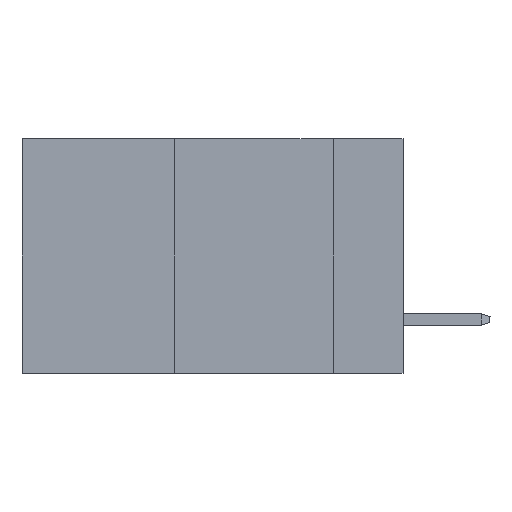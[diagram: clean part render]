
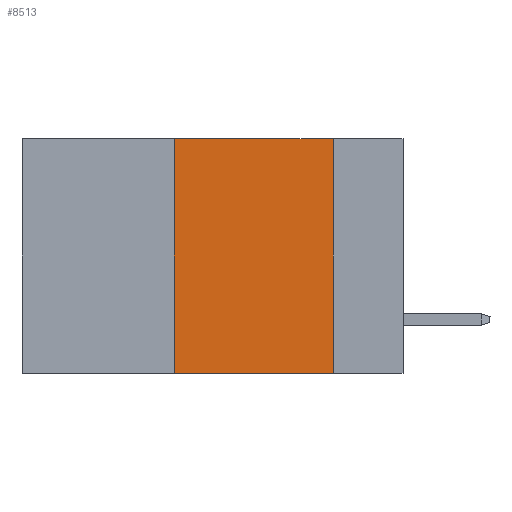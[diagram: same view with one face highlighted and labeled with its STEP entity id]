
A CAD part, left-side view. The second image highlights one B-rep face of the part: STEP entity #8513.
In plain terms, the highlighted planar face has unit normal (-1, 0, 0).
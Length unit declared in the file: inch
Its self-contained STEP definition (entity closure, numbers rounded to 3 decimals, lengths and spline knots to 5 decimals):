
#437 = EDGE_CURVE ( 'NONE', #2663, #17115, #24255, .T. ) ;
#637 = ORIENTED_EDGE ( 'NONE', *, *, #437, .F. ) ;
#1599 = ORIENTED_EDGE ( 'NONE', *, *, #24198, .F. ) ;
#2663 = VERTEX_POINT ( 'NONE', #20978 ) ;
#2784 = FACE_OUTER_BOUND ( 'NONE', #12183, .T. ) ;
#3086 = CARTESIAN_POINT ( 'NONE',  ( 0., 0.11, -0.37 ) ) ;
#4114 = VERTEX_POINT ( 'NONE', #3086 ) ;
#4499 = CARTESIAN_POINT ( 'NONE',  ( 0., 0.6, 0. ) ) ;
#4787 = LINE ( 'NONE', #12706, #25133 ) ;
#6580 = DIRECTION ( 'NONE',  ( 0., 0., -1. ) ) ;
#6811 = PLANE ( 'NONE',  #9851 ) ;
#7783 = LINE ( 'NONE', #20158, #24062 ) ;
#8513 = ADVANCED_FACE ( 'NONE', ( #2784 ), #6811, .F. ) ;
#8565 = DIRECTION ( 'NONE',  ( 0., -1., 0. ) ) ;
#8574 = DIRECTION ( 'NONE',  ( 0., 0., 1. ) ) ;
#9851 = AXIS2_PLACEMENT_3D ( 'NONE', #4499, #24205, #6580 ) ;
#10406 = CARTESIAN_POINT ( 'NONE',  ( 0., 0.36, 0. ) ) ;
#12183 = EDGE_LOOP ( 'NONE', ( #1599, #21915, #637, #22017 ) ) ;
#12706 = CARTESIAN_POINT ( 'NONE',  ( 0., 0.6, -0.37 ) ) ;
#13404 = VECTOR ( 'NONE', #8574, 39.37008 ) ;
#13510 = VECTOR ( 'NONE', #24924, 39.37008 ) ;
#13601 = EDGE_CURVE ( 'NONE', #17115, #19496, #7783, .T. ) ;
#14270 = CARTESIAN_POINT ( 'NONE',  ( 0., 0.36, 0. ) ) ;
#15670 = DIRECTION ( 'NONE',  ( 0., -1., 0. ) ) ;
#17115 = VERTEX_POINT ( 'NONE', #10406 ) ;
#18944 = LINE ( 'NONE', #22840, #13510 ) ;
#19496 = VERTEX_POINT ( 'NONE', #22279 ) ;
#20158 = CARTESIAN_POINT ( 'NONE',  ( 0., 0.6, 0. ) ) ;
#20978 = CARTESIAN_POINT ( 'NONE',  ( 0., 0.36, -0.37 ) ) ;
#21915 = ORIENTED_EDGE ( 'NONE', *, *, #13601, .F. ) ;
#22017 = ORIENTED_EDGE ( 'NONE', *, *, #24961, .T. ) ;
#22279 = CARTESIAN_POINT ( 'NONE',  ( 0., 0.11, 0. ) ) ;
#22840 = CARTESIAN_POINT ( 'NONE',  ( 0., 0.11, 0. ) ) ;
#24062 = VECTOR ( 'NONE', #15670, 39.37008 ) ;
#24198 = EDGE_CURVE ( 'NONE', #19496, #4114, #18944, .T. ) ;
#24205 = DIRECTION ( 'NONE',  ( 1., 0., 0. ) ) ;
#24255 = LINE ( 'NONE', #14270, #13404 ) ;
#24924 = DIRECTION ( 'NONE',  ( 0., 0., -1. ) ) ;
#24961 = EDGE_CURVE ( 'NONE', #2663, #4114, #4787, .T. ) ;
#25133 = VECTOR ( 'NONE', #8565, 39.37008 ) ;
